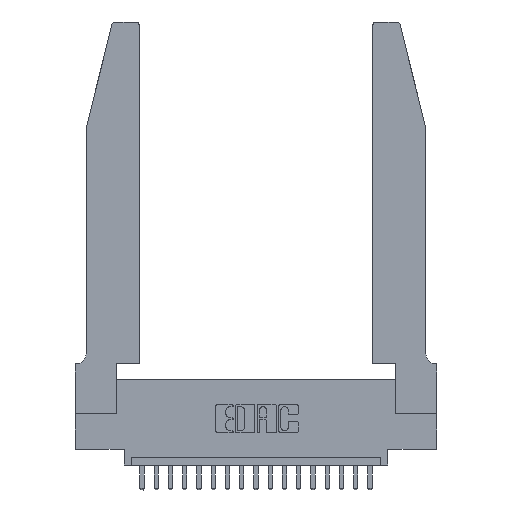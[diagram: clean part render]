
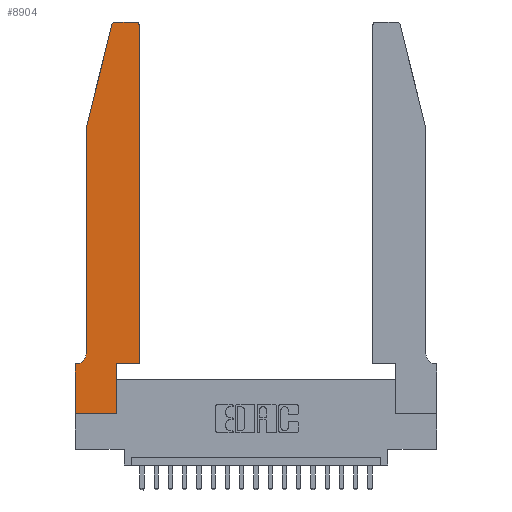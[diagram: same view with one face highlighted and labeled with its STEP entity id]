
A CAD part, top view. The second image highlights one B-rep face of the part: STEP entity #8904.
In plain terms, the highlighted planar face has unit normal (0, 0, 1).
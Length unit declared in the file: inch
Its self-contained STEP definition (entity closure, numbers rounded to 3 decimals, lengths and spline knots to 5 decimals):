
#37 = EDGE_CURVE ( 'NONE', #15818, #11451, #7531, .T. ) ;
#484 = CARTESIAN_POINT ( 'NONE',  ( 0.4505, 2.72, 0.37 ) ) ;
#640 = VECTOR ( 'NONE', #2965, 39.37008 ) ;
#718 = CARTESIAN_POINT ( 'NONE',  ( 0.25487, 2.72718, 0.37 ) ) ;
#752 = ORIENTED_EDGE ( 'NONE', *, *, #1457, .T. ) ;
#838 = CARTESIAN_POINT ( 'NONE',  ( 0., 0.35, 0.37 ) ) ;
#958 = ORIENTED_EDGE ( 'NONE', *, *, #16679, .T. ) ;
#1030 = DIRECTION ( 'NONE',  ( 0., -1., 0. ) ) ;
#1149 = CARTESIAN_POINT ( 'NONE',  ( 0.2865, 0.35, 0.37 ) ) ;
#1163 = DIRECTION ( 'NONE',  ( 1., 0., 0. ) ) ;
#1223 = CARTESIAN_POINT ( 'NONE',  ( 0.4505, 0.35, 0.37 ) ) ;
#1457 = EDGE_CURVE ( 'NONE', #9567, #14528, #6960, .T. ) ;
#1625 = DIRECTION ( 'NONE',  ( -0.239, -0.971, 0. ) ) ;
#1771 = ORIENTED_EDGE ( 'NONE', *, *, #5653, .T. ) ;
#2044 = VERTEX_POINT ( 'NONE', #11353 ) ;
#2506 = DIRECTION ( 'NONE',  ( 0., 0., 1. ) ) ;
#2901 = DIRECTION ( 'NONE',  ( 0., 0., 1. ) ) ;
#2965 = DIRECTION ( 'NONE',  ( 1., 0., 0. ) ) ;
#3210 = CARTESIAN_POINT ( 'NONE',  ( 0.0755, 2., 0.37 ) ) ;
#3432 = LINE ( 'NONE', #3210, #19211 ) ;
#3677 = DIRECTION ( 'NONE',  ( -1., 0., 0. ) ) ;
#4040 = DIRECTION ( 'NONE',  ( 1., 0., 0. ) ) ;
#4073 = ORIENTED_EDGE ( 'NONE', *, *, #7163, .T. ) ;
#4332 = VERTEX_POINT ( 'NONE', #17735 ) ;
#4544 = CARTESIAN_POINT ( 'NONE',  ( 0.284, 2.72, 0.37 ) ) ;
#4690 = ORIENTED_EDGE ( 'NONE', *, *, #18681, .T. ) ;
#4837 = DIRECTION ( 'NONE',  ( 0., 1., 0. ) ) ;
#5090 = CARTESIAN_POINT ( 'NONE',  ( 0.4205, 2.75, 0.37 ) ) ;
#5189 = ORIENTED_EDGE ( 'NONE', *, *, #13515, .T. ) ;
#5424 = EDGE_CURVE ( 'NONE', #5943, #10816, #11635, .T. ) ;
#5620 = EDGE_CURVE ( 'NONE', #16109, #5943, #9354, .T. ) ;
#5653 = EDGE_CURVE ( 'NONE', #12706, #15818, #17235, .T. ) ;
#5816 = DIRECTION ( 'NONE',  ( 1., 0., 0. ) ) ;
#5943 = VERTEX_POINT ( 'NONE', #484 ) ;
#6011 = CARTESIAN_POINT ( 'NONE',  ( 0.4505, 0.35, 0.37 ) ) ;
#6235 = LINE ( 'NONE', #7173, #14876 ) ;
#6785 = EDGE_CURVE ( 'NONE', #16525, #2044, #3432, .T. ) ;
#6835 = CARTESIAN_POINT ( 'NONE',  ( 0.0055, 0.42, 0.37 ) ) ;
#6960 = CIRCLE ( 'NONE', #19369, 0.07 ) ;
#7152 = ORIENTED_EDGE ( 'NONE', *, *, #37, .T. ) ;
#7163 = EDGE_CURVE ( 'NONE', #2044, #9567, #13596, .T. ) ;
#7173 = CARTESIAN_POINT ( 'NONE',  ( 0.2605, 2.75, 0.37 ) ) ;
#7531 = LINE ( 'NONE', #9089, #11081 ) ;
#7816 = LINE ( 'NONE', #1149, #17709 ) ;
#8057 = DIRECTION ( 'NONE',  ( -1., 0., 0. ) ) ;
#8479 = CARTESIAN_POINT ( 'NONE',  ( 0.2865, 0., 0.37 ) ) ;
#8546 = CARTESIAN_POINT ( 'NONE',  ( 0., 0.35, 0.37 ) ) ;
#8634 = VERTEX_POINT ( 'NONE', #17483 ) ;
#8687 = CARTESIAN_POINT ( 'NONE',  ( 0.0055, 0.35, 0.37 ) ) ;
#8904 = ADVANCED_FACE ( 'NONE', ( #11817 ), #10786, .T. ) ;
#9089 = CARTESIAN_POINT ( 'NONE',  ( 0., 0., 0.37 ) ) ;
#9258 = EDGE_CURVE ( 'NONE', #14528, #12706, #15870, .T. ) ;
#9354 = LINE ( 'NONE', #20360, #14706 ) ;
#9465 = ORIENTED_EDGE ( 'NONE', *, *, #5424, .T. ) ;
#9567 = VERTEX_POINT ( 'NONE', #19738 ) ;
#10786 = PLANE ( 'NONE',  #14416 ) ;
#10816 = VERTEX_POINT ( 'NONE', #5090 ) ;
#11026 = AXIS2_PLACEMENT_3D ( 'NONE', #4544, #19333, #17614 ) ;
#11081 = VECTOR ( 'NONE', #4040, 39.37008 ) ;
#11127 = ORIENTED_EDGE ( 'NONE', *, *, #6785, .T. ) ;
#11353 = CARTESIAN_POINT ( 'NONE',  ( 0.0755, 2., 0.37 ) ) ;
#11398 = CIRCLE ( 'NONE', #11026, 0.03 ) ;
#11451 = VERTEX_POINT ( 'NONE', #8479 ) ;
#11635 = CIRCLE ( 'NONE', #18051, 0.03 ) ;
#11725 = DIRECTION ( 'NONE',  ( 0., 0., -1. ) ) ;
#11774 = CARTESIAN_POINT ( 'NONE',  ( 0.0755, 2., 0.37 ) ) ;
#11817 = FACE_OUTER_BOUND ( 'NONE', #11982, .T. ) ;
#11982 = EDGE_LOOP ( 'NONE', ( #4690, #958, #11127, #4073, #752, #19149, #1771, #7152, #19724, #5189, #13156, #9465 ) ) ;
#12706 = VERTEX_POINT ( 'NONE', #8546 ) ;
#12731 = CARTESIAN_POINT ( 'NONE',  ( 0.0755, 0.35, 0.37 ) ) ;
#13156 = ORIENTED_EDGE ( 'NONE', *, *, #5620, .T. ) ;
#13515 = EDGE_CURVE ( 'NONE', #8634, #16109, #20024, .T. ) ;
#13575 = EDGE_CURVE ( 'NONE', #11451, #8634, #7816, .T. ) ;
#13596 = LINE ( 'NONE', #11774, #16383 ) ;
#14229 = CARTESIAN_POINT ( 'NONE',  ( 0.4205, 2.72, 0.37 ) ) ;
#14416 = AXIS2_PLACEMENT_3D ( 'NONE', #838, #2506, #5816 ) ;
#14528 = VERTEX_POINT ( 'NONE', #8687 ) ;
#14706 = VECTOR ( 'NONE', #15597, 39.37008 ) ;
#14876 = VECTOR ( 'NONE', #16806, 39.37008 ) ;
#15247 = CARTESIAN_POINT ( 'NONE',  ( 0., 0., 0.37 ) ) ;
#15597 = DIRECTION ( 'NONE',  ( 0., 1., 0. ) ) ;
#15818 = VERTEX_POINT ( 'NONE', #15247 ) ;
#15870 = LINE ( 'NONE', #12731, #19175 ) ;
#16109 = VERTEX_POINT ( 'NONE', #6011 ) ;
#16383 = VECTOR ( 'NONE', #1030, 39.37008 ) ;
#16459 = VECTOR ( 'NONE', #20811, 39.37008 ) ;
#16525 = VERTEX_POINT ( 'NONE', #718 ) ;
#16679 = EDGE_CURVE ( 'NONE', #4332, #16525, #11398, .T. ) ;
#16806 = DIRECTION ( 'NONE',  ( -1., 0., 0. ) ) ;
#17219 = CARTESIAN_POINT ( 'NONE',  ( 0., 0., 0.37 ) ) ;
#17235 = LINE ( 'NONE', #17219, #16459 ) ;
#17483 = CARTESIAN_POINT ( 'NONE',  ( 0.2865, 0.35, 0.37 ) ) ;
#17614 = DIRECTION ( 'NONE',  ( 1., 0., 0. ) ) ;
#17709 = VECTOR ( 'NONE', #4837, 39.37008 ) ;
#17735 = CARTESIAN_POINT ( 'NONE',  ( 0.284, 2.75, 0.37 ) ) ;
#18051 = AXIS2_PLACEMENT_3D ( 'NONE', #14229, #2901, #1163 ) ;
#18681 = EDGE_CURVE ( 'NONE', #10816, #4332, #6235, .T. ) ;
#19149 = ORIENTED_EDGE ( 'NONE', *, *, #9258, .T. ) ;
#19175 = VECTOR ( 'NONE', #8057, 39.37008 ) ;
#19211 = VECTOR ( 'NONE', #1625, 39.37008 ) ;
#19333 = DIRECTION ( 'NONE',  ( 0., 0., 1. ) ) ;
#19369 = AXIS2_PLACEMENT_3D ( 'NONE', #6835, #11725, #3677 ) ;
#19724 = ORIENTED_EDGE ( 'NONE', *, *, #13575, .T. ) ;
#19738 = CARTESIAN_POINT ( 'NONE',  ( 0.0755, 0.42, 0.37 ) ) ;
#20024 = LINE ( 'NONE', #1223, #640 ) ;
#20360 = CARTESIAN_POINT ( 'NONE',  ( 0.4505, 0.35, 0.37 ) ) ;
#20811 = DIRECTION ( 'NONE',  ( 0., -1., 0. ) ) ;
